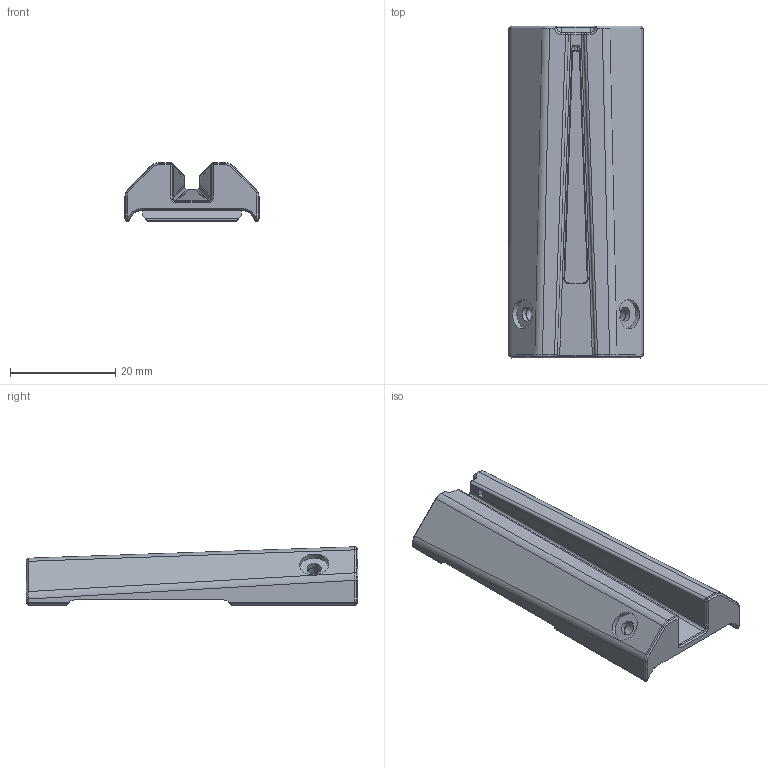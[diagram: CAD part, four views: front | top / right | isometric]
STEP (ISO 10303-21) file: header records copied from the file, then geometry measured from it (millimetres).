
FILE_DESCRIPTION(/* description */ (''),/* implementation_level */ '2;1');
FILE_NAME(/* name */ 'Guttersnipe Sight.step',/* time_stamp */ '2021-06-23T20:35:04-04:00',/* author */ (''),/* organization */ (''),/* preprocessor_version */ 'ST-DEVELOPER v18.1',/* originating_system */ 'Autodesk Translation Framework v10.9.0.1377',/* authorisation */ '');
FILE_SCHEMA (('AUTOMOTIVE_DESIGN { 1 0 10303 214 3 1 1 }'));
Length unit declared in the file: millimetre
Products named in the file (1): Guttersnipe Sight
Bounding box: 25.5 x 63.1 x 11.1 mm (x, y, z)
Volume: 7044.2 mm3; surface area: 9685.6 mm2
Topology: 5 solids, 7 shells, 562 faces, 1357 edges, 804 vertices
Faces by surface type: plane 193, bspline 158, cylinder 139, cone 54, torus 12, sphere 6
Full cylindrical faces by diameter (mm): 2.7 x3, 5.6 x2
Entity records: 18767 total; most frequent: CARTESIAN_POINT 6446, ORIENTED_EDGE 2690, DIRECTION 2334, EDGE_CURVE 1345, AXIS2_PLACEMENT_3D 838, VERTEX_POINT 804, LINE 658, VECTOR 658
